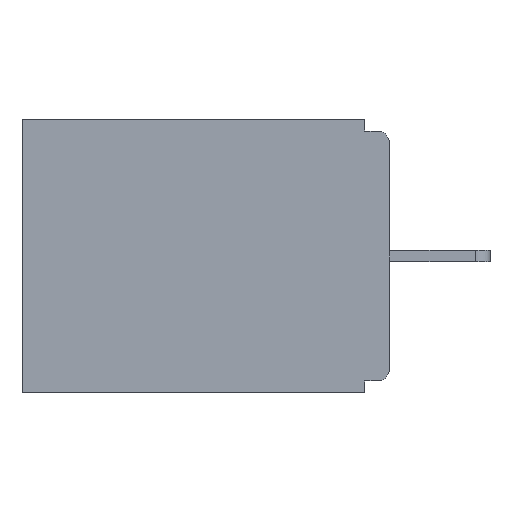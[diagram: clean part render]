
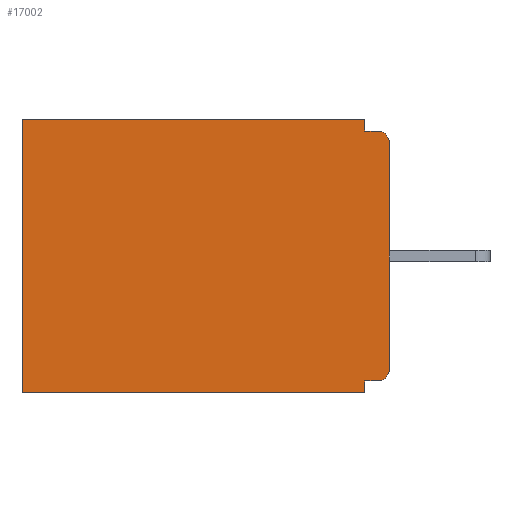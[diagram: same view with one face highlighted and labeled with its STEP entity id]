
A CAD part, left-side view. The second image highlights one B-rep face of the part: STEP entity #17002.
In plain terms, the highlighted planar face has unit normal (-1, 0, 0).
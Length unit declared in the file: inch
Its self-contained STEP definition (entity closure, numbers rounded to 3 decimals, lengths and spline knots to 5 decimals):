
#25 = CARTESIAN_POINT ( 'NONE',  ( 0.298, 0.015, -0.03 ) ) ;
#53 = VERTEX_POINT ( 'NONE', #13357 ) ;
#109 = DIRECTION ( 'NONE',  ( 0., 1., 0. ) ) ;
#458 = CARTESIAN_POINT ( 'NONE',  ( 0.298, 0., -0.343 ) ) ;
#976 = CARTESIAN_POINT ( 'NONE',  ( 0.298, 0.031, -0.343 ) ) ;
#1409 = DIRECTION ( 'NONE',  ( 0., 0., -1. ) ) ;
#1700 = CARTESIAN_POINT ( 'NONE',  ( 0.298, 0.031, -0.015 ) ) ;
#1720 = ORIENTED_EDGE ( 'NONE', *, *, #4446, .F. ) ;
#1818 = CARTESIAN_POINT ( 'NONE',  ( 0.298, 0., 0. ) ) ;
#2024 = ORIENTED_EDGE ( 'NONE', *, *, #12200, .F. ) ;
#2089 = CIRCLE ( 'NONE', #10881, 0.015 ) ;
#2252 = EDGE_LOOP ( 'NONE', ( #9068, #1720, #2024, #9137, #6461, #7291, #14527, #13954, #14938, #4773 ) ) ;
#2434 = CARTESIAN_POINT ( 'NONE',  ( 0.298, 0.015, -0.015 ) ) ;
#2789 = CARTESIAN_POINT ( 'NONE',  ( 0.298, 0.031, -0.328 ) ) ;
#3106 = EDGE_CURVE ( 'NONE', #3905, #5860, #10743, .T. ) ;
#3195 = DIRECTION ( 'NONE',  ( 0., 0., -1. ) ) ;
#3266 = VECTOR ( 'NONE', #4479, 39.37008 ) ;
#3549 = LINE ( 'NONE', #7610, #10688 ) ;
#3648 = CARTESIAN_POINT ( 'NONE',  ( 0.298, 0.46, -0.343 ) ) ;
#3762 = CARTESIAN_POINT ( 'NONE',  ( 0.298, 0.015, -0.313 ) ) ;
#3905 = VERTEX_POINT ( 'NONE', #10455 ) ;
#4422 = LINE ( 'NONE', #458, #14585 ) ;
#4446 = EDGE_CURVE ( 'NONE', #15199, #8565, #3549, .T. ) ;
#4479 = DIRECTION ( 'NONE',  ( 0., 0., -1. ) ) ;
#4773 = ORIENTED_EDGE ( 'NONE', *, *, #9758, .F. ) ;
#4899 = VECTOR ( 'NONE', #109, 39.37008 ) ;
#5146 = DIRECTION ( 'NONE',  ( 0., 0., -1. ) ) ;
#5259 = VERTEX_POINT ( 'NONE', #2789 ) ;
#5860 = VERTEX_POINT ( 'NONE', #8618 ) ;
#5951 = VERTEX_POINT ( 'NONE', #16346 ) ;
#5981 = CARTESIAN_POINT ( 'NONE',  ( 0.298, 0., 0. ) ) ;
#6337 = DIRECTION ( 'NONE',  ( 0., 0., -1. ) ) ;
#6461 = ORIENTED_EDGE ( 'NONE', *, *, #9732, .T. ) ;
#6892 = LINE ( 'NONE', #8494, #3266 ) ;
#7239 = PLANE ( 'NONE',  #11483 ) ;
#7291 = ORIENTED_EDGE ( 'NONE', *, *, #8941, .F. ) ;
#7358 = DIRECTION ( 'NONE',  ( 0., 1., 0. ) ) ;
#7592 = CARTESIAN_POINT ( 'NONE',  ( 0.298, 0.46, 0. ) ) ;
#7610 = CARTESIAN_POINT ( 'NONE',  ( 0.298, 0., -0.015 ) ) ;
#7754 = EDGE_CURVE ( 'NONE', #9930, #5259, #9506, .T. ) ;
#8061 = VERTEX_POINT ( 'NONE', #3648 ) ;
#8360 = CARTESIAN_POINT ( 'NONE',  ( 0.298, 0.031, -0.343 ) ) ;
#8494 = CARTESIAN_POINT ( 'NONE',  ( 0.298, 0.031, -0.343 ) ) ;
#8565 = VERTEX_POINT ( 'NONE', #2434 ) ;
#8618 = CARTESIAN_POINT ( 'NONE',  ( 0.298, 0.46, 0. ) ) ;
#8658 = AXIS2_PLACEMENT_3D ( 'NONE', #25, #9517, #1409 ) ;
#8706 = LINE ( 'NONE', #976, #12624 ) ;
#8908 = DIRECTION ( 'NONE',  ( 0., 0., -1. ) ) ;
#8923 = CARTESIAN_POINT ( 'NONE',  ( 0.298, 0., -0.328 ) ) ;
#8941 = EDGE_CURVE ( 'NONE', #11201, #8061, #4422, .T. ) ;
#8952 = CIRCLE ( 'NONE', #8658, 0.015 ) ;
#8997 = VECTOR ( 'NONE', #6337, 39.37008 ) ;
#9068 = ORIENTED_EDGE ( 'NONE', *, *, #11784, .T. ) ;
#9081 = VECTOR ( 'NONE', #7358, 39.37008 ) ;
#9093 = DIRECTION ( 'NONE',  ( 0., 0., -1. ) ) ;
#9137 = ORIENTED_EDGE ( 'NONE', *, *, #3106, .T. ) ;
#9417 = VECTOR ( 'NONE', #8908, 39.37008 ) ;
#9506 = LINE ( 'NONE', #8923, #9081 ) ;
#9517 = DIRECTION ( 'NONE',  ( -1., 0., 0. ) ) ;
#9732 = EDGE_CURVE ( 'NONE', #5860, #8061, #16327, .T. ) ;
#9758 = EDGE_CURVE ( 'NONE', #5951, #53, #15525, .T. ) ;
#9930 = VERTEX_POINT ( 'NONE', #14583 ) ;
#10455 = CARTESIAN_POINT ( 'NONE',  ( 0.298, 0.031, 0. ) ) ;
#10688 = VECTOR ( 'NONE', #13096, 39.37008 ) ;
#10743 = LINE ( 'NONE', #5981, #4899 ) ;
#10881 = AXIS2_PLACEMENT_3D ( 'NONE', #3762, #13109, #5146 ) ;
#11201 = VERTEX_POINT ( 'NONE', #8360 ) ;
#11239 = DIRECTION ( 'NONE',  ( 1., 0., 0. ) ) ;
#11483 = AXIS2_PLACEMENT_3D ( 'NONE', #1818, #11239, #3195 ) ;
#11784 = EDGE_CURVE ( 'NONE', #5951, #8565, #8952, .T. ) ;
#12200 = EDGE_CURVE ( 'NONE', #3905, #15199, #8706, .T. ) ;
#12466 = FACE_OUTER_BOUND ( 'NONE', #2252, .T. ) ;
#12624 = VECTOR ( 'NONE', #9093, 39.37008 ) ;
#12840 = EDGE_CURVE ( 'NONE', #9930, #53, #2089, .T. ) ;
#13096 = DIRECTION ( 'NONE',  ( 0., -1., 0. ) ) ;
#13109 = DIRECTION ( 'NONE',  ( -1., 0., 0. ) ) ;
#13357 = CARTESIAN_POINT ( 'NONE',  ( 0.298, 0., -0.313 ) ) ;
#13954 = ORIENTED_EDGE ( 'NONE', *, *, #7754, .F. ) ;
#14236 = CARTESIAN_POINT ( 'NONE',  ( 0.298, 0., 0. ) ) ;
#14527 = ORIENTED_EDGE ( 'NONE', *, *, #16332, .F. ) ;
#14583 = CARTESIAN_POINT ( 'NONE',  ( 0.298, 0.015, -0.328 ) ) ;
#14585 = VECTOR ( 'NONE', #15123, 39.37008 ) ;
#14938 = ORIENTED_EDGE ( 'NONE', *, *, #12840, .T. ) ;
#15123 = DIRECTION ( 'NONE',  ( 0., 1., 0. ) ) ;
#15199 = VERTEX_POINT ( 'NONE', #1700 ) ;
#15525 = LINE ( 'NONE', #14236, #8997 ) ;
#16327 = LINE ( 'NONE', #7592, #9417 ) ;
#16332 = EDGE_CURVE ( 'NONE', #5259, #11201, #6892, .T. ) ;
#16346 = CARTESIAN_POINT ( 'NONE',  ( 0.298, 0., -0.03 ) ) ;
#17002 = ADVANCED_FACE ( 'NONE', ( #12466 ), #7239, .F. ) ;
